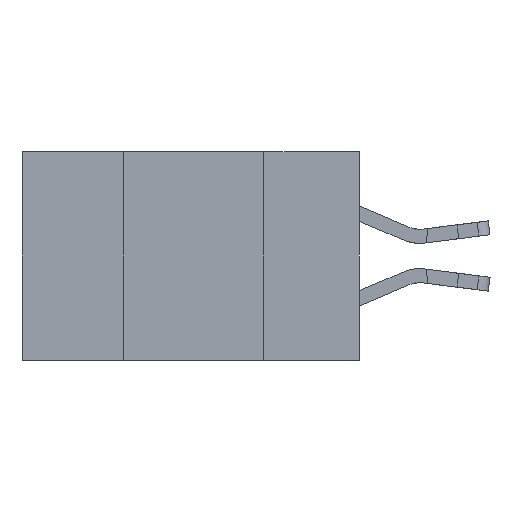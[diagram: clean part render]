
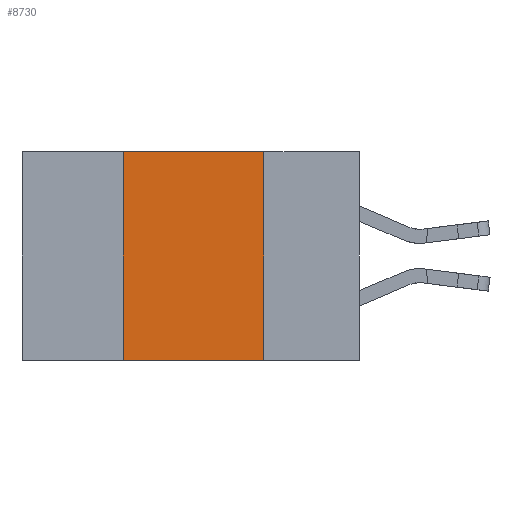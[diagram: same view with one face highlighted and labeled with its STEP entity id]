
A CAD part, left-side view. The second image highlights one B-rep face of the part: STEP entity #8730.
In plain terms, the highlighted planar face has unit normal (-1, 0, 0).
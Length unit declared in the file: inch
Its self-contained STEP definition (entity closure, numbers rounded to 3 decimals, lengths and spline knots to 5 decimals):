
#1236 = EDGE_LOOP ( 'NONE', ( #25735, #7673, #6819, #11279 ) ) ;
#3768 = DIRECTION ( 'NONE',  ( 0., 0., -1. ) ) ;
#4087 = VECTOR ( 'NONE', #23722, 39.37008 ) ;
#5234 = LINE ( 'NONE', #14257, #4087 ) ;
#5914 = DIRECTION ( 'NONE',  ( 1., 0., 0. ) ) ;
#5928 = CARTESIAN_POINT ( 'NONE',  ( 0., 0.42, -0.37 ) ) ;
#6248 = VERTEX_POINT ( 'NONE', #20839 ) ;
#6363 = CARTESIAN_POINT ( 'NONE',  ( 0., 0.42, 0. ) ) ;
#6819 = ORIENTED_EDGE ( 'NONE', *, *, #21744, .F. ) ;
#7673 = ORIENTED_EDGE ( 'NONE', *, *, #19475, .F. ) ;
#7757 = EDGE_CURVE ( 'NONE', #6248, #7842, #17179, .T. ) ;
#7842 = VERTEX_POINT ( 'NONE', #12944 ) ;
#8730 = ADVANCED_FACE ( 'NONE', ( #10674 ), #18306, .F. ) ;
#9255 = LINE ( 'NONE', #22743, #17580 ) ;
#10674 = FACE_OUTER_BOUND ( 'NONE', #1236, .T. ) ;
#11279 = ORIENTED_EDGE ( 'NONE', *, *, #27346, .T. ) ;
#12276 = CARTESIAN_POINT ( 'NONE',  ( 0., 0.17, 0. ) ) ;
#12944 = CARTESIAN_POINT ( 'NONE',  ( 0., 0.17, -0.37 ) ) ;
#14257 = CARTESIAN_POINT ( 'NONE',  ( 0., 0.6, 0. ) ) ;
#15410 = DIRECTION ( 'NONE',  ( 0., -1., 0. ) ) ;
#15540 = LINE ( 'NONE', #30653, #16296 ) ;
#16296 = VECTOR ( 'NONE', #20979, 39.37008 ) ;
#17179 = LINE ( 'NONE', #12276, #22909 ) ;
#17580 = VECTOR ( 'NONE', #15410, 39.37008 ) ;
#18306 = PLANE ( 'NONE',  #28810 ) ;
#19475 = EDGE_CURVE ( 'NONE', #22510, #6248, #5234, .T. ) ;
#20765 = CARTESIAN_POINT ( 'NONE',  ( 0., 0.6, 0. ) ) ;
#20839 = CARTESIAN_POINT ( 'NONE',  ( 0., 0.17, 0. ) ) ;
#20979 = DIRECTION ( 'NONE',  ( 0., 0., 1. ) ) ;
#21744 = EDGE_CURVE ( 'NONE', #24296, #22510, #15540, .T. ) ;
#22510 = VERTEX_POINT ( 'NONE', #6363 ) ;
#22743 = CARTESIAN_POINT ( 'NONE',  ( 0., 0.6, -0.37 ) ) ;
#22909 = VECTOR ( 'NONE', #24503, 39.37008 ) ;
#23722 = DIRECTION ( 'NONE',  ( 0., -1., 0. ) ) ;
#24296 = VERTEX_POINT ( 'NONE', #5928 ) ;
#24503 = DIRECTION ( 'NONE',  ( 0., 0., -1. ) ) ;
#25735 = ORIENTED_EDGE ( 'NONE', *, *, #7757, .F. ) ;
#27346 = EDGE_CURVE ( 'NONE', #24296, #7842, #9255, .T. ) ;
#28810 = AXIS2_PLACEMENT_3D ( 'NONE', #20765, #5914, #3768 ) ;
#30653 = CARTESIAN_POINT ( 'NONE',  ( 0., 0.42, 0. ) ) ;
